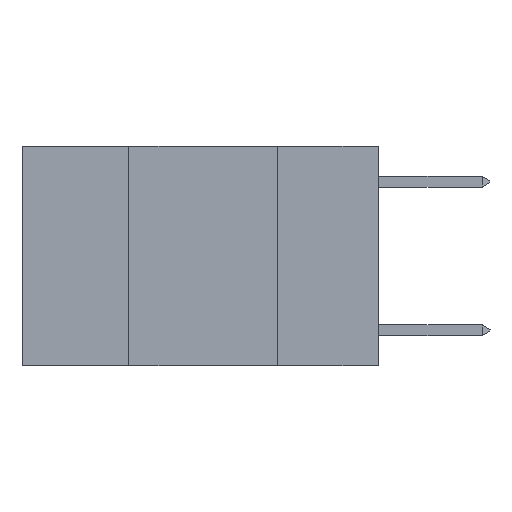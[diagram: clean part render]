
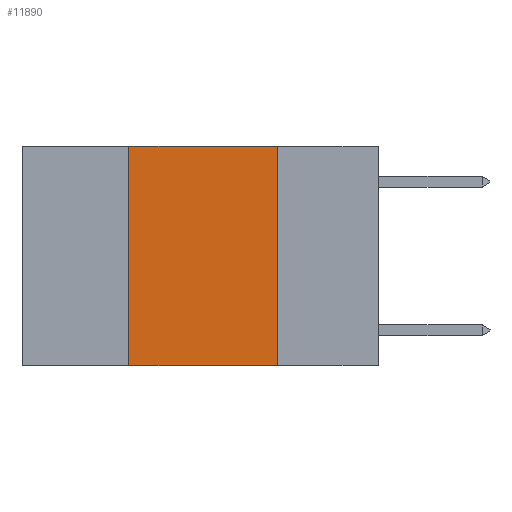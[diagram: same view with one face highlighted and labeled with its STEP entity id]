
A CAD part, left-side view. The second image highlights one B-rep face of the part: STEP entity #11890.
In plain terms, the highlighted planar face has unit normal (-1, 0, 0).
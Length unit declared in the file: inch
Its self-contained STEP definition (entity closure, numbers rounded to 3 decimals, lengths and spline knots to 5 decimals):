
#935 = VERTEX_POINT ( 'NONE', #7368 ) ;
#3788 = DIRECTION ( 'NONE',  ( 0., -1., 0. ) ) ;
#4283 = DIRECTION ( 'NONE',  ( 0., 0., -1. ) ) ;
#7368 = CARTESIAN_POINT ( 'NONE',  ( 0., 0.42, 0. ) ) ;
#7475 = VERTEX_POINT ( 'NONE', #16180 ) ;
#7967 = CARTESIAN_POINT ( 'NONE',  ( 0., 0.6, 0. ) ) ;
#8276 = LINE ( 'NONE', #15026, #8456 ) ;
#8456 = VECTOR ( 'NONE', #3788, 39.37008 ) ;
#8980 = DIRECTION ( 'NONE',  ( 1., 0., 0. ) ) ;
#9151 = DIRECTION ( 'NONE',  ( 0., 0., -1. ) ) ;
#9572 = CARTESIAN_POINT ( 'NONE',  ( 0., 0.42, 0. ) ) ;
#9626 = CARTESIAN_POINT ( 'NONE',  ( 0., 0.6, 0. ) ) ;
#9894 = PLANE ( 'NONE',  #21596 ) ;
#9907 = DIRECTION ( 'NONE',  ( 0., -1., 0. ) ) ;
#11339 = ORIENTED_EDGE ( 'NONE', *, *, #14388, .F. ) ;
#11491 = VERTEX_POINT ( 'NONE', #23290 ) ;
#11733 = VERTEX_POINT ( 'NONE', #14804 ) ;
#11890 = ADVANCED_FACE ( 'NONE', ( #20947 ), #9894, .F. ) ;
#11945 = ORIENTED_EDGE ( 'NONE', *, *, #20764, .F. ) ;
#11972 = ORIENTED_EDGE ( 'NONE', *, *, #16823, .F. ) ;
#12582 = ORIENTED_EDGE ( 'NONE', *, *, #19104, .T. ) ;
#12819 = VECTOR ( 'NONE', #13254, 39.37008 ) ;
#13071 = LINE ( 'NONE', #9572, #12819 ) ;
#13254 = DIRECTION ( 'NONE',  ( 0., 0., 1. ) ) ;
#13656 = CARTESIAN_POINT ( 'NONE',  ( 0., 0.17, 0. ) ) ;
#14388 = EDGE_CURVE ( 'NONE', #7475, #11491, #17446, .T. ) ;
#14804 = CARTESIAN_POINT ( 'NONE',  ( 0., 0.42, -0.37 ) ) ;
#15026 = CARTESIAN_POINT ( 'NONE',  ( 0., 0.6, -0.37 ) ) ;
#16180 = CARTESIAN_POINT ( 'NONE',  ( 0., 0.17, 0. ) ) ;
#16823 = EDGE_CURVE ( 'NONE', #11733, #935, #13071, .T. ) ;
#16874 = VECTOR ( 'NONE', #9907, 39.37008 ) ;
#17311 = VECTOR ( 'NONE', #4283, 39.37008 ) ;
#17378 = LINE ( 'NONE', #7967, #16874 ) ;
#17446 = LINE ( 'NONE', #13656, #17311 ) ;
#18196 = EDGE_LOOP ( 'NONE', ( #11339, #11945, #11972, #12582 ) ) ;
#19104 = EDGE_CURVE ( 'NONE', #11733, #11491, #8276, .T. ) ;
#20764 = EDGE_CURVE ( 'NONE', #935, #7475, #17378, .T. ) ;
#20947 = FACE_OUTER_BOUND ( 'NONE', #18196, .T. ) ;
#21596 = AXIS2_PLACEMENT_3D ( 'NONE', #9626, #8980, #9151 ) ;
#23290 = CARTESIAN_POINT ( 'NONE',  ( 0., 0.17, -0.37 ) ) ;
